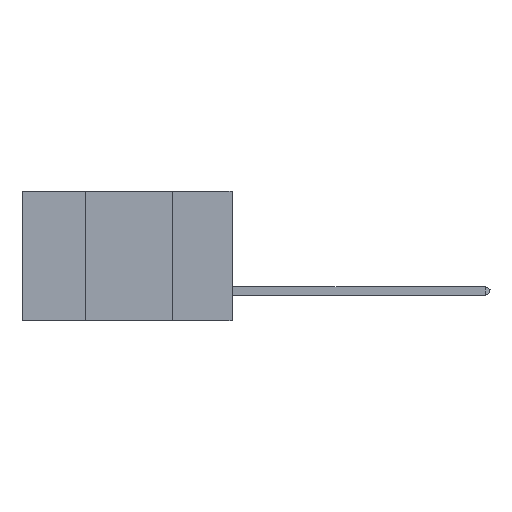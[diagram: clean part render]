
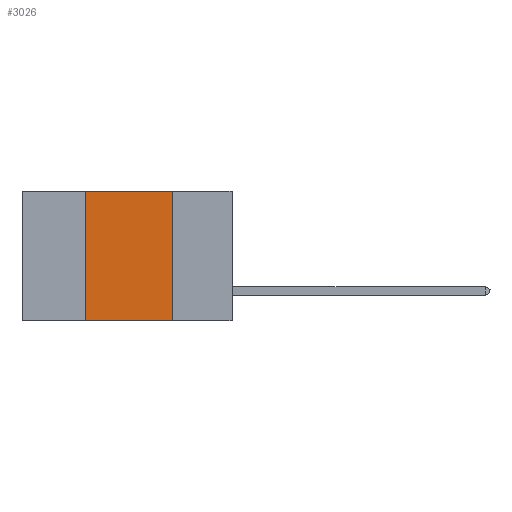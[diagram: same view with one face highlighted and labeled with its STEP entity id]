
A CAD part, left-side view. The second image highlights one B-rep face of the part: STEP entity #3026.
In plain terms, the highlighted planar face has unit normal (-1, 0, 0).
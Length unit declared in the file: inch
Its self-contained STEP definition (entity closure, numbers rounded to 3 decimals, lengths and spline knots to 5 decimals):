
#1953 = VERTEX_POINT ( 'NONE', #18525 ) ;
#3026 = ADVANCED_FACE ( 'NONE', ( #22309 ), #32568, .F. ) ;
#3820 = CARTESIAN_POINT ( 'NONE',  ( 0., 0.6, 0. ) ) ;
#3926 = CARTESIAN_POINT ( 'NONE',  ( 0., 0.17, 0. ) ) ;
#4089 = VERTEX_POINT ( 'NONE', #19291 ) ;
#6250 = VECTOR ( 'NONE', #6855, 39.37008 ) ;
#6632 = ORIENTED_EDGE ( 'NONE', *, *, #28450, .T. ) ;
#6855 = DIRECTION ( 'NONE',  ( 0., -1., 0. ) ) ;
#7474 = LINE ( 'NONE', #16456, #25128 ) ;
#8771 = DIRECTION ( 'NONE',  ( 0., 0., -1. ) ) ;
#9144 = ORIENTED_EDGE ( 'NONE', *, *, #32200, .F. ) ;
#12241 = EDGE_CURVE ( 'NONE', #1953, #20026, #20295, .T. ) ;
#12595 = DIRECTION ( 'NONE',  ( 0., -1., 0. ) ) ;
#13174 = LINE ( 'NONE', #30241, #24430 ) ;
#13992 = DIRECTION ( 'NONE',  ( 0., 0., 1. ) ) ;
#14910 = DIRECTION ( 'NONE',  ( 0., 0., -1. ) ) ;
#15364 = AXIS2_PLACEMENT_3D ( 'NONE', #22341, #30183, #14910 ) ;
#16296 = ORIENTED_EDGE ( 'NONE', *, *, #18395, .F. ) ;
#16456 = CARTESIAN_POINT ( 'NONE',  ( 0., 0.42, 0. ) ) ;
#17538 = LINE ( 'NONE', #3926, #25961 ) ;
#18395 = EDGE_CURVE ( 'NONE', #20026, #4089, #17538, .T. ) ;
#18525 = CARTESIAN_POINT ( 'NONE',  ( 0., 0.42, 0. ) ) ;
#19291 = CARTESIAN_POINT ( 'NONE',  ( 0., 0.17, -0.37 ) ) ;
#20026 = VERTEX_POINT ( 'NONE', #22164 ) ;
#20295 = LINE ( 'NONE', #3820, #6250 ) ;
#20633 = CARTESIAN_POINT ( 'NONE',  ( 0., 0.42, -0.37 ) ) ;
#22164 = CARTESIAN_POINT ( 'NONE',  ( 0., 0.17, 0. ) ) ;
#22309 = FACE_OUTER_BOUND ( 'NONE', #31722, .T. ) ;
#22341 = CARTESIAN_POINT ( 'NONE',  ( 0., 0.6, 0. ) ) ;
#23034 = ORIENTED_EDGE ( 'NONE', *, *, #12241, .F. ) ;
#23745 = VERTEX_POINT ( 'NONE', #20633 ) ;
#24430 = VECTOR ( 'NONE', #12595, 39.37008 ) ;
#25128 = VECTOR ( 'NONE', #13992, 39.37008 ) ;
#25961 = VECTOR ( 'NONE', #8771, 39.37008 ) ;
#28450 = EDGE_CURVE ( 'NONE', #23745, #4089, #13174, .T. ) ;
#30183 = DIRECTION ( 'NONE',  ( 1., 0., 0. ) ) ;
#30241 = CARTESIAN_POINT ( 'NONE',  ( 0., 0.6, -0.37 ) ) ;
#31722 = EDGE_LOOP ( 'NONE', ( #16296, #23034, #9144, #6632 ) ) ;
#32200 = EDGE_CURVE ( 'NONE', #23745, #1953, #7474, .T. ) ;
#32568 = PLANE ( 'NONE',  #15364 ) ;
